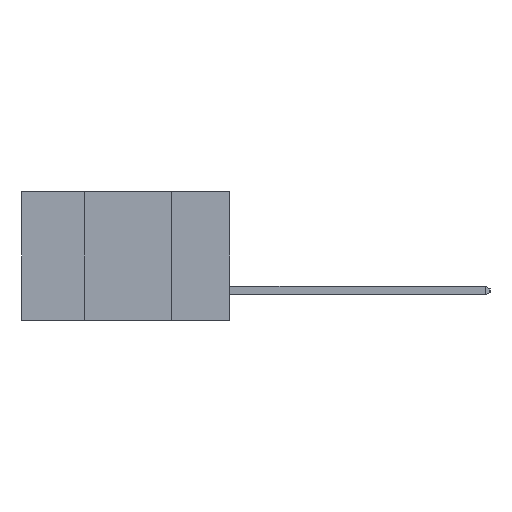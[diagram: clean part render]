
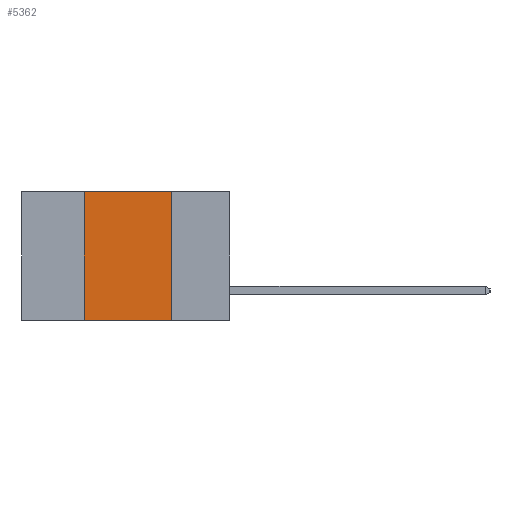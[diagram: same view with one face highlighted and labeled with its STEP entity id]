
A CAD part, left-side view. The second image highlights one B-rep face of the part: STEP entity #5362.
In plain terms, the highlighted planar face has unit normal (-1, 0, 0).
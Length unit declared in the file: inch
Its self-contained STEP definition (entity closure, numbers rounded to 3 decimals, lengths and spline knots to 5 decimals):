
#302 = AXIS2_PLACEMENT_3D ( 'NONE', #8611, #8638, #8736 ) ;
#660 = CARTESIAN_POINT ( 'NONE',  ( 0., 0.17, -0.37 ) ) ;
#1744 = DIRECTION ( 'NONE',  ( 0., 0., 1. ) ) ;
#1821 = VERTEX_POINT ( 'NONE', #8006 ) ;
#1982 = CARTESIAN_POINT ( 'NONE',  ( 0., 0.42, -0.37 ) ) ;
#2335 = CARTESIAN_POINT ( 'NONE',  ( 0., 0.17, -0.37 ) ) ;
#3124 = LINE ( 'NONE', #1982, #7866 ) ;
#3771 = VERTEX_POINT ( 'NONE', #21364 ) ;
#5362 = ADVANCED_FACE ( 'NONE', ( #9232 ), #9299, .F. ) ;
#5889 = LINE ( 'NONE', #660, #9995 ) ;
#6647 = ORIENTED_EDGE ( 'NONE', *, *, #10384, .F. ) ;
#7554 = LINE ( 'NONE', #10802, #16698 ) ;
#7866 = VECTOR ( 'NONE', #1744, 39.37008 ) ;
#8006 = CARTESIAN_POINT ( 'NONE',  ( 0., 0.17, 0. ) ) ;
#8253 = CARTESIAN_POINT ( 'NONE',  ( 0., 0.42, 0. ) ) ;
#8611 = CARTESIAN_POINT ( 'NONE',  ( 0., 0.6, 0. ) ) ;
#8638 = DIRECTION ( 'NONE',  ( 1., 0., 0. ) ) ;
#8736 = DIRECTION ( 'NONE',  ( 0., 0., -1. ) ) ;
#9232 = FACE_OUTER_BOUND ( 'NONE', #11546, .T. ) ;
#9299 = PLANE ( 'NONE',  #302 ) ;
#9995 = VECTOR ( 'NONE', #11302, 39.37008 ) ;
#10384 = EDGE_CURVE ( 'NONE', #15932, #1821, #14374, .T. ) ;
#10428 = CARTESIAN_POINT ( 'NONE',  ( 0., 0.6, 0. ) ) ;
#10802 = CARTESIAN_POINT ( 'NONE',  ( 0., 0.6, -0.37 ) ) ;
#10863 = DIRECTION ( 'NONE',  ( 0., -1., 0. ) ) ;
#10937 = DIRECTION ( 'NONE',  ( 0., -1., 0. ) ) ;
#11082 = VERTEX_POINT ( 'NONE', #2335 ) ;
#11302 = DIRECTION ( 'NONE',  ( 0., 0., -1. ) ) ;
#11374 = EDGE_CURVE ( 'NONE', #3771, #11082, #7554, .T. ) ;
#11546 = EDGE_LOOP ( 'NONE', ( #21967, #6647, #11857, #20731 ) ) ;
#11857 = ORIENTED_EDGE ( 'NONE', *, *, #13257, .F. ) ;
#13257 = EDGE_CURVE ( 'NONE', #3771, #15932, #3124, .T. ) ;
#13836 = VECTOR ( 'NONE', #10937, 39.37008 ) ;
#14374 = LINE ( 'NONE', #10428, #13836 ) ;
#14388 = EDGE_CURVE ( 'NONE', #1821, #11082, #5889, .T. ) ;
#15932 = VERTEX_POINT ( 'NONE', #8253 ) ;
#16698 = VECTOR ( 'NONE', #10863, 39.37008 ) ;
#20731 = ORIENTED_EDGE ( 'NONE', *, *, #11374, .T. ) ;
#21364 = CARTESIAN_POINT ( 'NONE',  ( 0., 0.42, -0.37 ) ) ;
#21967 = ORIENTED_EDGE ( 'NONE', *, *, #14388, .F. ) ;
